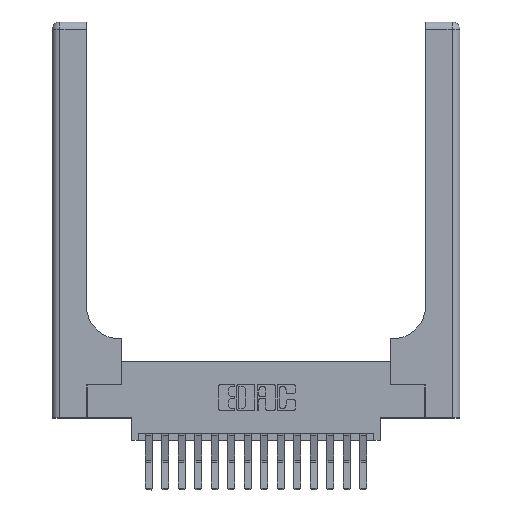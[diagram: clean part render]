
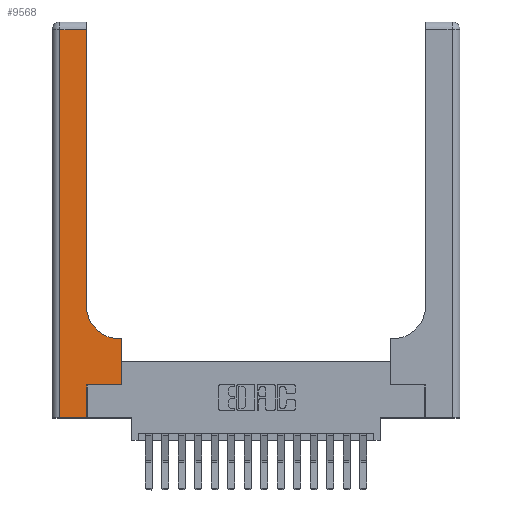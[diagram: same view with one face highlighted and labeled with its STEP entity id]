
A CAD part, top view. The second image highlights one B-rep face of the part: STEP entity #9568.
In plain terms, the highlighted planar face has unit normal (0, 0, 1).
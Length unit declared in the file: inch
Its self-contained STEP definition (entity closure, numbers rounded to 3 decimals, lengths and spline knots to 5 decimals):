
#296 = DIRECTION ( 'NONE',  ( -1., 0., 0. ) ) ;
#631 = CARTESIAN_POINT ( 'NONE',  ( 0., 2.94, 0.37 ) ) ;
#914 = CARTESIAN_POINT ( 'NONE',  ( 0.265, 0., 0.37 ) ) ;
#1037 = CARTESIAN_POINT ( 'NONE',  ( 0.06, 0., 0.37 ) ) ;
#1180 = VERTEX_POINT ( 'NONE', #13623 ) ;
#1936 = VECTOR ( 'NONE', #10891, 39.37008 ) ;
#2194 = CARTESIAN_POINT ( 'NONE',  ( 0.51, 0.6, 0.37 ) ) ;
#2457 = LINE ( 'NONE', #4740, #13315 ) ;
#2728 = EDGE_CURVE ( 'NONE', #3702, #9459, #9335, .T. ) ;
#3007 = DIRECTION ( 'NONE',  ( 0., 1., 0. ) ) ;
#3117 = ORIENTED_EDGE ( 'NONE', *, *, #15384, .T. ) ;
#3158 = CARTESIAN_POINT ( 'NONE',  ( 0., 3., 0.37 ) ) ;
#3210 = ORIENTED_EDGE ( 'NONE', *, *, #7561, .T. ) ;
#3323 = VECTOR ( 'NONE', #4685, 39.37008 ) ;
#3360 = CARTESIAN_POINT ( 'NONE',  ( 0.265, 0.25, 0.37 ) ) ;
#3702 = VERTEX_POINT ( 'NONE', #5071 ) ;
#4433 = CARTESIAN_POINT ( 'NONE',  ( 0.26, 0.85, 0.37 ) ) ;
#4621 = CARTESIAN_POINT ( 'NONE',  ( 0.26, 2.94, 0.37 ) ) ;
#4685 = DIRECTION ( 'NONE',  ( -1., 0., 0. ) ) ;
#4740 = CARTESIAN_POINT ( 'NONE',  ( 0.26, 3., 0.37 ) ) ;
#5071 = CARTESIAN_POINT ( 'NONE',  ( 0.528, 0.25, 0.37 ) ) ;
#5183 = EDGE_CURVE ( 'NONE', #8392, #17025, #18193, .T. ) ;
#5447 = DIRECTION ( 'NONE',  ( 0., 0., -1. ) ) ;
#5521 = CARTESIAN_POINT ( 'NONE',  ( 0.06, 2.94, 0.37 ) ) ;
#6208 = VECTOR ( 'NONE', #14834, 39.37008 ) ;
#6519 = CARTESIAN_POINT ( 'NONE',  ( 0.06, 3., 0.37 ) ) ;
#6974 = EDGE_LOOP ( 'NONE', ( #3210, #3117, #11183, #17371, #8584, #17533, #15258, #17126, #14059 ) ) ;
#7561 = EDGE_CURVE ( 'NONE', #17025, #17755, #2457, .T. ) ;
#8392 = VERTEX_POINT ( 'NONE', #2194 ) ;
#8584 = ORIENTED_EDGE ( 'NONE', *, *, #10325, .T. ) ;
#8903 = EDGE_CURVE ( 'NONE', #1180, #3702, #12411, .T. ) ;
#8927 = DIRECTION ( 'NONE',  ( 0., 0., -1. ) ) ;
#8988 = VERTEX_POINT ( 'NONE', #15082 ) ;
#9121 = LINE ( 'NONE', #914, #1936 ) ;
#9266 = DIRECTION ( 'NONE',  ( 0., -1., 0. ) ) ;
#9335 = LINE ( 'NONE', #11508, #16729 ) ;
#9459 = VERTEX_POINT ( 'NONE', #12754 ) ;
#9568 = ADVANCED_FACE ( 'NONE', ( #9785 ), #17257, .F. ) ;
#9785 = FACE_OUTER_BOUND ( 'NONE', #6974, .T. ) ;
#9836 = LINE ( 'NONE', #12549, #13110 ) ;
#9975 = LINE ( 'NONE', #631, #6208 ) ;
#10325 = EDGE_CURVE ( 'NONE', #8988, #1180, #9121, .T. ) ;
#10891 = DIRECTION ( 'NONE',  ( 0., 1., 0. ) ) ;
#11183 = ORIENTED_EDGE ( 'NONE', *, *, #15060, .T. ) ;
#11207 = AXIS2_PLACEMENT_3D ( 'NONE', #3158, #8927, #296 ) ;
#11508 = CARTESIAN_POINT ( 'NONE',  ( 0.528, 0.25, 0.37 ) ) ;
#11519 = LINE ( 'NONE', #6519, #15214 ) ;
#11730 = CARTESIAN_POINT ( 'NONE',  ( 0.26, 0.6, 0.37 ) ) ;
#11780 = DIRECTION ( 'NONE',  ( 0., 1., 0. ) ) ;
#12411 = LINE ( 'NONE', #3360, #15699 ) ;
#12549 = CARTESIAN_POINT ( 'NONE',  ( 0., 0., 0.37 ) ) ;
#12754 = CARTESIAN_POINT ( 'NONE',  ( 0.528, 0.6, 0.37 ) ) ;
#13110 = VECTOR ( 'NONE', #16762, 39.37008 ) ;
#13280 = EDGE_CURVE ( 'NONE', #15172, #8988, #9836, .T. ) ;
#13315 = VECTOR ( 'NONE', #11780, 39.37008 ) ;
#13623 = CARTESIAN_POINT ( 'NONE',  ( 0.265, 0.25, 0.37 ) ) ;
#13884 = CARTESIAN_POINT ( 'NONE',  ( 0.51, 0.85, 0.37 ) ) ;
#14059 = ORIENTED_EDGE ( 'NONE', *, *, #5183, .T. ) ;
#14661 = DIRECTION ( 'NONE',  ( 1., 0., 0. ) ) ;
#14834 = DIRECTION ( 'NONE',  ( -1., 0., 0. ) ) ;
#15060 = EDGE_CURVE ( 'NONE', #16336, #15172, #11519, .T. ) ;
#15082 = CARTESIAN_POINT ( 'NONE',  ( 0.265, 0., 0.37 ) ) ;
#15172 = VERTEX_POINT ( 'NONE', #1037 ) ;
#15214 = VECTOR ( 'NONE', #9266, 39.37008 ) ;
#15258 = ORIENTED_EDGE ( 'NONE', *, *, #2728, .T. ) ;
#15273 = DIRECTION ( 'NONE',  ( 1., 0., 0. ) ) ;
#15384 = EDGE_CURVE ( 'NONE', #17755, #16336, #9975, .T. ) ;
#15699 = VECTOR ( 'NONE', #14661, 39.37008 ) ;
#16336 = VERTEX_POINT ( 'NONE', #5521 ) ;
#16622 = AXIS2_PLACEMENT_3D ( 'NONE', #13884, #5447, #15273 ) ;
#16729 = VECTOR ( 'NONE', #3007, 39.37008 ) ;
#16762 = DIRECTION ( 'NONE',  ( 1., 0., 0. ) ) ;
#17025 = VERTEX_POINT ( 'NONE', #4433 ) ;
#17126 = ORIENTED_EDGE ( 'NONE', *, *, #17142, .T. ) ;
#17142 = EDGE_CURVE ( 'NONE', #9459, #8392, #18296, .T. ) ;
#17257 = PLANE ( 'NONE',  #11207 ) ;
#17371 = ORIENTED_EDGE ( 'NONE', *, *, #13280, .T. ) ;
#17533 = ORIENTED_EDGE ( 'NONE', *, *, #8903, .T. ) ;
#17755 = VERTEX_POINT ( 'NONE', #4621 ) ;
#18193 = CIRCLE ( 'NONE', #16622, 0.25 ) ;
#18296 = LINE ( 'NONE', #11730, #3323 ) ;
